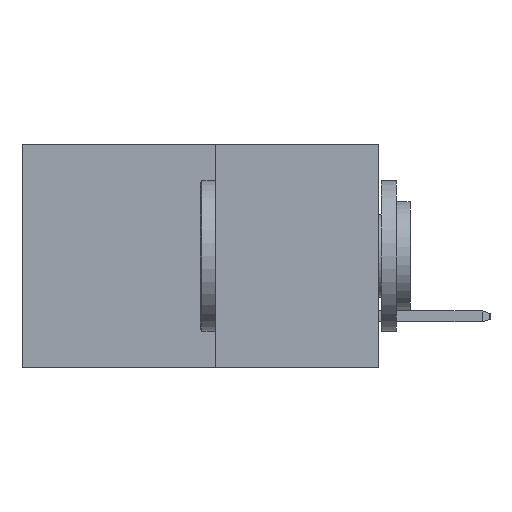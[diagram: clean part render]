
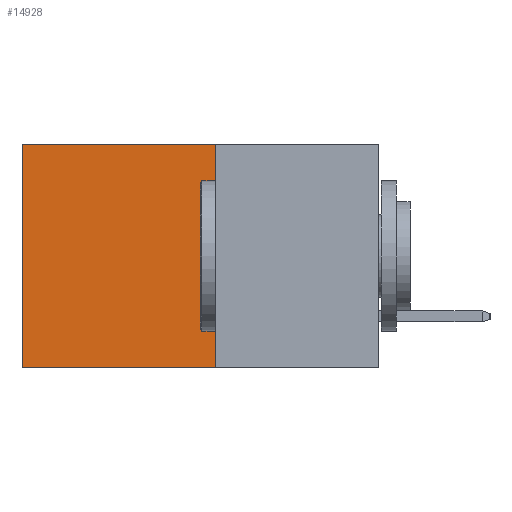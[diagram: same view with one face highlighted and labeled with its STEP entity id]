
A CAD part, left-side view. The second image highlights one B-rep face of the part: STEP entity #14928.
In plain terms, the highlighted planar face has unit normal (-1, 0, 0).
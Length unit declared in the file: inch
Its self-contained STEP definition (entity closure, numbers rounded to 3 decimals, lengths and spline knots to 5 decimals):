
#2306 = VECTOR ( 'NONE', #22980, 39.37008 ) ;
#3170 = VECTOR ( 'NONE', #21032, 39.37008 ) ;
#4144 = CARTESIAN_POINT ( 'NONE',  ( 0.277, 0.27, -0.37 ) ) ;
#4329 = CARTESIAN_POINT ( 'NONE',  ( 0.277, 0.27, -0.37 ) ) ;
#4466 = VERTEX_POINT ( 'NONE', #17580 ) ;
#5030 = VERTEX_POINT ( 'NONE', #4144 ) ;
#5509 = LINE ( 'NONE', #11374, #10581 ) ;
#6375 = ORIENTED_EDGE ( 'NONE', *, *, #14452, .T. ) ;
#6521 = DIRECTION ( 'NONE',  ( 1., 0., 0. ) ) ;
#8093 = LINE ( 'NONE', #20867, #2306 ) ;
#8260 = EDGE_CURVE ( 'NONE', #14528, #9823, #26814, .T. ) ;
#8615 = PLANE ( 'NONE',  #17980 ) ;
#8960 = LINE ( 'NONE', #23057, #3170 ) ;
#9823 = VERTEX_POINT ( 'NONE', #11077 ) ;
#9889 = VECTOR ( 'NONE', #11083, 39.37008 ) ;
#10581 = VECTOR ( 'NONE', #19857, 39.37008 ) ;
#11077 = CARTESIAN_POINT ( 'NONE',  ( 0.277, 0.59, -0.37 ) ) ;
#11083 = DIRECTION ( 'NONE',  ( 0., 0., -1. ) ) ;
#11163 = ORIENTED_EDGE ( 'NONE', *, *, #18807, .F. ) ;
#11374 = CARTESIAN_POINT ( 'NONE',  ( 0.277, 0.27, -0.37 ) ) ;
#14452 = EDGE_CURVE ( 'NONE', #4466, #14528, #8960, .T. ) ;
#14528 = VERTEX_POINT ( 'NONE', #27553 ) ;
#14706 = EDGE_LOOP ( 'NONE', ( #21295, #11163, #16505, #6375 ) ) ;
#14928 = ADVANCED_FACE ( 'NONE', ( #18276 ), #8615, .F. ) ;
#16505 = ORIENTED_EDGE ( 'NONE', *, *, #25708, .F. ) ;
#17580 = CARTESIAN_POINT ( 'NONE',  ( 0.277, 0.27, 0. ) ) ;
#17980 = AXIS2_PLACEMENT_3D ( 'NONE', #4329, #6521, #21441 ) ;
#18276 = FACE_OUTER_BOUND ( 'NONE', #14706, .T. ) ;
#18807 = EDGE_CURVE ( 'NONE', #5030, #9823, #8093, .T. ) ;
#19857 = DIRECTION ( 'NONE',  ( 0., 0., -1. ) ) ;
#20867 = CARTESIAN_POINT ( 'NONE',  ( 0.277, 0.27, -0.37 ) ) ;
#21032 = DIRECTION ( 'NONE',  ( 0., 1., 0. ) ) ;
#21295 = ORIENTED_EDGE ( 'NONE', *, *, #8260, .T. ) ;
#21441 = DIRECTION ( 'NONE',  ( 0., 0., -1. ) ) ;
#21662 = CARTESIAN_POINT ( 'NONE',  ( 0.277, 0.59, -0.37 ) ) ;
#22980 = DIRECTION ( 'NONE',  ( 0., 1., 0. ) ) ;
#23057 = CARTESIAN_POINT ( 'NONE',  ( 0.277, 0.27, 0. ) ) ;
#25708 = EDGE_CURVE ( 'NONE', #4466, #5030, #5509, .T. ) ;
#26814 = LINE ( 'NONE', #21662, #9889 ) ;
#27553 = CARTESIAN_POINT ( 'NONE',  ( 0.277, 0.59, 0. ) ) ;
